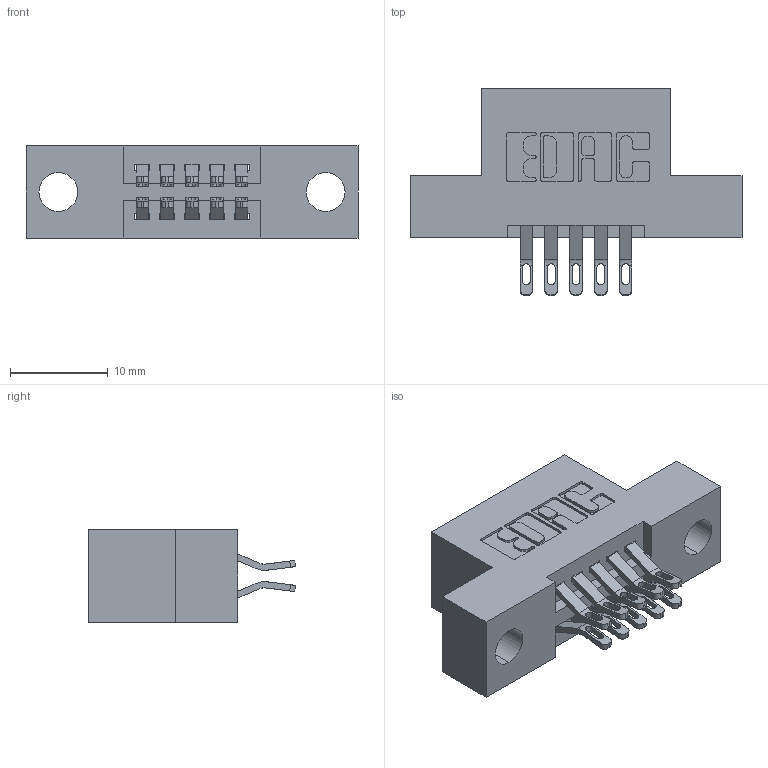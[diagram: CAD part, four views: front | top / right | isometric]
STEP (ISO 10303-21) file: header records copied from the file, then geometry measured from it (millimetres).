
FILE_DESCRIPTION (( 'STEP AP203' ), '1' );
FILE_NAME ('395-010-555-204.STEP', '2021-06-14T17:26:58', ( '' ), ( '' ), 'SwSTEP 2.0', 'SolidWorks 2020', '' );
FILE_SCHEMA (( 'CONFIG_CONTROL_DESIGN' ));
Length unit declared in the file: inch
Products named in the file (3): 395-010-555-204; 345-292-001_555 Tail; 345 Part_Flush Mounting Lugs - 0.156 Dia-TI
Assembly tree (11 placements, depth 2):
  395-010-555-204
    345 Part_Flush Mounting Lugs - 0.156 Dia-TI
    345-292-001_555 Tail  x10
Bounding box: 33.91 x 21.13 x 9.4 mm (x, y, z)
Volume: 2873.6 mm3; surface area: 3483.5 mm2
Topology: 11 solids, 11 shells, 700 faces, 2147 edges, 1430 vertices
Faces by surface type: plane 404, cylinder 296
Entity records: 9649 total; most frequent: CARTESIAN_POINT 1692, ORIENTED_EDGE 1594, DIRECTION 1505, EDGE_CURVE 797, LINE 625, VECTOR 625, VERTEX_POINT 530, AXIS2_PLACEMENT_3D 440
